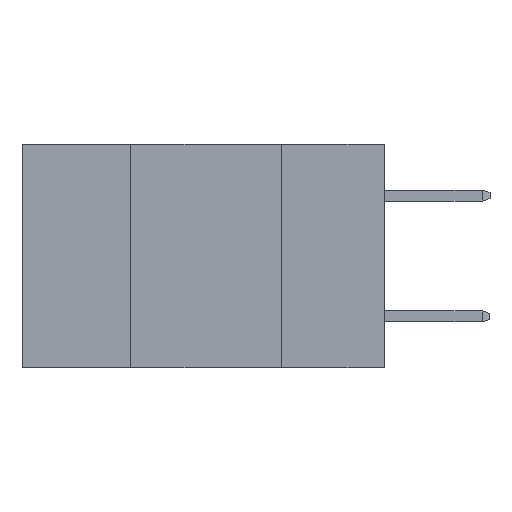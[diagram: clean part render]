
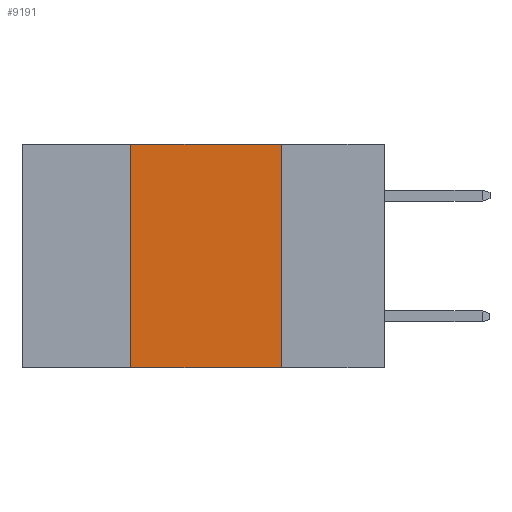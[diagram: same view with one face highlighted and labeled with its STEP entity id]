
A CAD part, left-side view. The second image highlights one B-rep face of the part: STEP entity #9191.
In plain terms, the highlighted planar face has unit normal (-1, 0, 0).
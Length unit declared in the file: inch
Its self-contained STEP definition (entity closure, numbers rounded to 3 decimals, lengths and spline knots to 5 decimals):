
#53 = EDGE_CURVE ( 'NONE', #1644, #9353, #12002, .T. ) ;
#878 = EDGE_CURVE ( 'NONE', #1644, #17645, #10300, .T. ) ;
#1644 = VERTEX_POINT ( 'NONE', #4768 ) ;
#2196 = PLANE ( 'NONE',  #21897 ) ;
#2837 = VECTOR ( 'NONE', #23346, 39.37008 ) ;
#3528 = CARTESIAN_POINT ( 'NONE',  ( 0., 0.17, 0. ) ) ;
#4073 = DIRECTION ( 'NONE',  ( 1., 0., 0. ) ) ;
#4768 = CARTESIAN_POINT ( 'NONE',  ( 0., 0.42, -0.37 ) ) ;
#5904 = VECTOR ( 'NONE', #13045, 39.37008 ) ;
#6170 = EDGE_LOOP ( 'NONE', ( #22601, #18394, #23151, #14706 ) ) ;
#6335 = CARTESIAN_POINT ( 'NONE',  ( 0., 0.6, -0.37 ) ) ;
#6666 = FACE_OUTER_BOUND ( 'NONE', #6170, .T. ) ;
#7455 = DIRECTION ( 'NONE',  ( 0., -1., 0. ) ) ;
#7781 = LINE ( 'NONE', #12606, #2837 ) ;
#7800 = CARTESIAN_POINT ( 'NONE',  ( 0., 0.17, -0.37 ) ) ;
#8881 = EDGE_CURVE ( 'NONE', #18493, #17645, #12474, .T. ) ;
#9083 = CARTESIAN_POINT ( 'NONE',  ( 0., 0.17, 0. ) ) ;
#9191 = ADVANCED_FACE ( 'NONE', ( #6666 ), #2196, .F. ) ;
#9353 = VERTEX_POINT ( 'NONE', #22661 ) ;
#9567 = EDGE_CURVE ( 'NONE', #9353, #18493, #7781, .T. ) ;
#10300 = LINE ( 'NONE', #6335, #19342 ) ;
#12002 = LINE ( 'NONE', #13526, #5904 ) ;
#12474 = LINE ( 'NONE', #3528, #18386 ) ;
#12606 = CARTESIAN_POINT ( 'NONE',  ( 0., 0.6, 0. ) ) ;
#13045 = DIRECTION ( 'NONE',  ( 0., 0., 1. ) ) ;
#13526 = CARTESIAN_POINT ( 'NONE',  ( 0., 0.42, 0. ) ) ;
#14706 = ORIENTED_EDGE ( 'NONE', *, *, #878, .T. ) ;
#15105 = CARTESIAN_POINT ( 'NONE',  ( 0., 0.6, 0. ) ) ;
#16357 = DIRECTION ( 'NONE',  ( 0., 0., -1. ) ) ;
#16886 = DIRECTION ( 'NONE',  ( 0., 0., -1. ) ) ;
#17645 = VERTEX_POINT ( 'NONE', #7800 ) ;
#18386 = VECTOR ( 'NONE', #16357, 39.37008 ) ;
#18394 = ORIENTED_EDGE ( 'NONE', *, *, #9567, .F. ) ;
#18493 = VERTEX_POINT ( 'NONE', #9083 ) ;
#19342 = VECTOR ( 'NONE', #7455, 39.37008 ) ;
#21897 = AXIS2_PLACEMENT_3D ( 'NONE', #15105, #4073, #16886 ) ;
#22601 = ORIENTED_EDGE ( 'NONE', *, *, #8881, .F. ) ;
#22661 = CARTESIAN_POINT ( 'NONE',  ( 0., 0.42, 0. ) ) ;
#23151 = ORIENTED_EDGE ( 'NONE', *, *, #53, .F. ) ;
#23346 = DIRECTION ( 'NONE',  ( 0., -1., 0. ) ) ;
